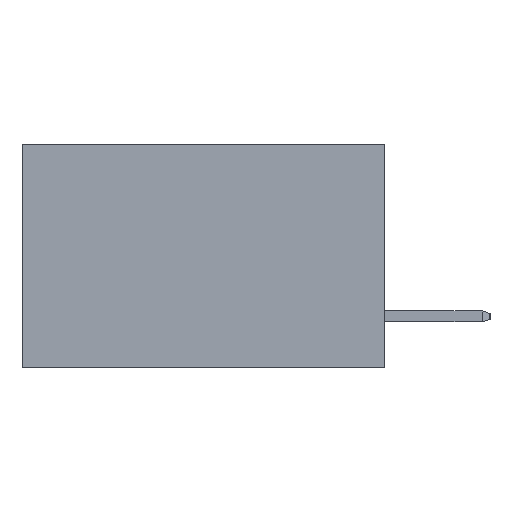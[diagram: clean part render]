
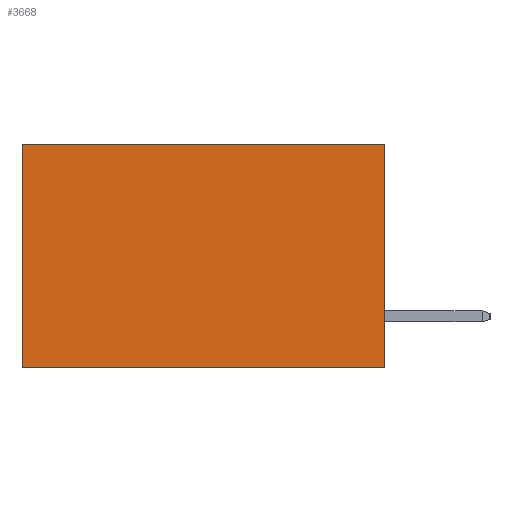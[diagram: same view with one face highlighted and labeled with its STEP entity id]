
A CAD part, left-side view. The second image highlights one B-rep face of the part: STEP entity #3668.
In plain terms, the highlighted planar face has unit normal (-1, 0, 0).
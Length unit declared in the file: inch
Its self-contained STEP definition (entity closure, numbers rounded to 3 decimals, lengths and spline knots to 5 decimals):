
#212 = ORIENTED_EDGE ( 'NONE', *, *, #7286, .T. ) ;
#269 = AXIS2_PLACEMENT_3D ( 'NONE', #5532, #3391, #4116 ) ;
#324 = LINE ( 'NONE', #1723, #4392 ) ;
#685 = ORIENTED_EDGE ( 'NONE', *, *, #7566, .T. ) ;
#909 = EDGE_LOOP ( 'NONE', ( #212, #5214, #6243, #685 ) ) ;
#1369 = CARTESIAN_POINT ( 'NONE',  ( 0.2615, 0., -0.37 ) ) ;
#1723 = CARTESIAN_POINT ( 'NONE',  ( 0.2615, 0.6, -0.37 ) ) ;
#2074 = CARTESIAN_POINT ( 'NONE',  ( 0.2615, 0.6, 0. ) ) ;
#2086 = LINE ( 'NONE', #8474, #9526 ) ;
#2202 = LINE ( 'NONE', #8914, #7901 ) ;
#2206 = VERTEX_POINT ( 'NONE', #2074 ) ;
#2476 = DIRECTION ( 'NONE',  ( 0., 0., -1. ) ) ;
#2969 = PLANE ( 'NONE',  #269 ) ;
#3298 = FACE_OUTER_BOUND ( 'NONE', #909, .T. ) ;
#3380 = CARTESIAN_POINT ( 'NONE',  ( 0.2615, 0.6, -0.37 ) ) ;
#3391 = DIRECTION ( 'NONE',  ( 1., 0., 0. ) ) ;
#3394 = VERTEX_POINT ( 'NONE', #1369 ) ;
#3418 = EDGE_CURVE ( 'NONE', #6558, #3394, #4438, .T. ) ;
#3668 = ADVANCED_FACE ( 'NONE', ( #3298 ), #2969, .F. ) ;
#4116 = DIRECTION ( 'NONE',  ( 0., 0., -1. ) ) ;
#4347 = DIRECTION ( 'NONE',  ( 0., 1., 0. ) ) ;
#4392 = VECTOR ( 'NONE', #2476, 39.37008 ) ;
#4438 = LINE ( 'NONE', #9334, #6133 ) ;
#4795 = DIRECTION ( 'NONE',  ( 0., 1., 0. ) ) ;
#5214 = ORIENTED_EDGE ( 'NONE', *, *, #8072, .F. ) ;
#5532 = CARTESIAN_POINT ( 'NONE',  ( 0.2615, 0., -0.37 ) ) ;
#6133 = VECTOR ( 'NONE', #9449, 39.37008 ) ;
#6243 = ORIENTED_EDGE ( 'NONE', *, *, #3418, .F. ) ;
#6558 = VERTEX_POINT ( 'NONE', #8398 ) ;
#7286 = EDGE_CURVE ( 'NONE', #2206, #9063, #324, .T. ) ;
#7566 = EDGE_CURVE ( 'NONE', #6558, #2206, #2086, .T. ) ;
#7901 = VECTOR ( 'NONE', #4795, 39.37008 ) ;
#8072 = EDGE_CURVE ( 'NONE', #3394, #9063, #2202, .T. ) ;
#8398 = CARTESIAN_POINT ( 'NONE',  ( 0.2615, 0., 0. ) ) ;
#8474 = CARTESIAN_POINT ( 'NONE',  ( 0.2615, 0., 0. ) ) ;
#8914 = CARTESIAN_POINT ( 'NONE',  ( 0.2615, 0., -0.37 ) ) ;
#9063 = VERTEX_POINT ( 'NONE', #3380 ) ;
#9334 = CARTESIAN_POINT ( 'NONE',  ( 0.2615, 0., -0.37 ) ) ;
#9449 = DIRECTION ( 'NONE',  ( 0., 0., -1. ) ) ;
#9526 = VECTOR ( 'NONE', #4347, 39.37008 ) ;
